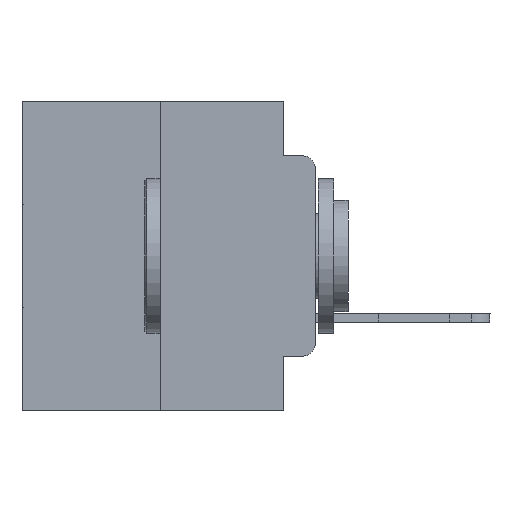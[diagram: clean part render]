
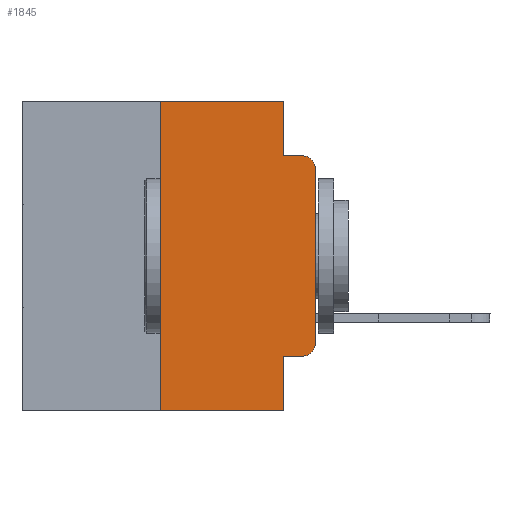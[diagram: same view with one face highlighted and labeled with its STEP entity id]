
A CAD part, left-side view. The second image highlights one B-rep face of the part: STEP entity #1845.
In plain terms, the highlighted planar face has unit normal (-1, 0, 0).
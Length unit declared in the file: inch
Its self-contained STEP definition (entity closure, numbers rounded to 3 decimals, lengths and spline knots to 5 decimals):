
#11 = VECTOR ( 'NONE', #9029, 39.37008 ) ;
#549 = ORIENTED_EDGE ( 'NONE', *, *, #20635, .T. ) ;
#1133 = VERTEX_POINT ( 'NONE', #3323 ) ;
#1257 = LINE ( 'NONE', #24410, #22145 ) ;
#1786 = CARTESIAN_POINT ( 'NONE',  ( 0., 0.02, -0.3915 ) ) ;
#1845 = ADVANCED_FACE ( 'NONE', ( #3311 ), #5530, .F. ) ;
#2125 = EDGE_CURVE ( 'NONE', #24953, #6071, #23184, .T. ) ;
#2326 = CARTESIAN_POINT ( 'NONE',  ( 0., 0.051, -0.0885 ) ) ;
#2658 = EDGE_CURVE ( 'NONE', #4916, #24879, #10917, .T. ) ;
#3274 = CARTESIAN_POINT ( 'NONE',  ( 0., 0.051, -0.5 ) ) ;
#3311 = FACE_OUTER_BOUND ( 'NONE', #5650, .T. ) ;
#3323 = CARTESIAN_POINT ( 'NONE',  ( 0., 0., -0.1085 ) ) ;
#3436 = CARTESIAN_POINT ( 'NONE',  ( 0., 0.051, 0. ) ) ;
#3917 = VERTEX_POINT ( 'NONE', #7481 ) ;
#4213 = CARTESIAN_POINT ( 'NONE',  ( 0., 0.473, 0. ) ) ;
#4224 = DIRECTION ( 'NONE',  ( 0., 0., 1. ) ) ;
#4415 = CARTESIAN_POINT ( 'NONE',  ( 0., 0., 0. ) ) ;
#4502 = CARTESIAN_POINT ( 'NONE',  ( 0., 0.02, -0.0885 ) ) ;
#4613 = EDGE_CURVE ( 'NONE', #24413, #24953, #23400, .T. ) ;
#4916 = VERTEX_POINT ( 'NONE', #19216 ) ;
#5120 = ORIENTED_EDGE ( 'NONE', *, *, #14701, .T. ) ;
#5386 = LINE ( 'NONE', #20365, #8354 ) ;
#5530 = PLANE ( 'NONE',  #8370 ) ;
#5650 = EDGE_LOOP ( 'NONE', ( #13415, #8074, #25949, #16573, #19299, #25915, #549, #20449, #17535, #5120 ) ) ;
#5832 = CIRCLE ( 'NONE', #15003, 0.02 ) ;
#6071 = VERTEX_POINT ( 'NONE', #3436 ) ;
#6528 = CIRCLE ( 'NONE', #19536, 0.02 ) ;
#6769 = VERTEX_POINT ( 'NONE', #2326 ) ;
#7481 = CARTESIAN_POINT ( 'NONE',  ( 0., 0.02, -0.4115 ) ) ;
#7547 = DIRECTION ( 'NONE',  ( 0., 0., -1. ) ) ;
#7846 = DIRECTION ( 'NONE',  ( 0., 0., -1. ) ) ;
#7897 = DIRECTION ( 'NONE',  ( -1., 0., 0. ) ) ;
#8070 = EDGE_CURVE ( 'NONE', #4916, #3917, #1257, .T. ) ;
#8074 = ORIENTED_EDGE ( 'NONE', *, *, #18147, .T. ) ;
#8200 = CARTESIAN_POINT ( 'NONE',  ( 0., 0.25, 0. ) ) ;
#8354 = VECTOR ( 'NONE', #7547, 39.37008 ) ;
#8370 = AXIS2_PLACEMENT_3D ( 'NONE', #14064, #20655, #7846 ) ;
#8768 = DIRECTION ( 'NONE',  ( 0., 0., -1. ) ) ;
#9029 = DIRECTION ( 'NONE',  ( 0., 0., -1. ) ) ;
#9088 = CARTESIAN_POINT ( 'NONE',  ( 0., 0., -0.3915 ) ) ;
#10396 = VECTOR ( 'NONE', #23461, 39.37008 ) ;
#10467 = VECTOR ( 'NONE', #21643, 39.37008 ) ;
#10805 = VECTOR ( 'NONE', #4224, 39.37008 ) ;
#10917 = LINE ( 'NONE', #19531, #11 ) ;
#11549 = CARTESIAN_POINT ( 'NONE',  ( 0., 0.25, -0.5 ) ) ;
#12240 = VECTOR ( 'NONE', #15158, 39.37008 ) ;
#12473 = LINE ( 'NONE', #4415, #10467 ) ;
#13415 = ORIENTED_EDGE ( 'NONE', *, *, #15674, .T. ) ;
#14064 = CARTESIAN_POINT ( 'NONE',  ( 0., 0.473, 0. ) ) ;
#14701 = EDGE_CURVE ( 'NONE', #3917, #21515, #5832, .T. ) ;
#15003 = AXIS2_PLACEMENT_3D ( 'NONE', #1786, #7897, #18744 ) ;
#15090 = DIRECTION ( 'NONE',  ( -1., 0., 0. ) ) ;
#15158 = DIRECTION ( 'NONE',  ( 0., -1., 0. ) ) ;
#15455 = CARTESIAN_POINT ( 'NONE',  ( 0., 0.02, -0.1085 ) ) ;
#15674 = EDGE_CURVE ( 'NONE', #21515, #1133, #12473, .T. ) ;
#15690 = DIRECTION ( 'NONE',  ( 0., -1., 0. ) ) ;
#16573 = ORIENTED_EDGE ( 'NONE', *, *, #22687, .F. ) ;
#16865 = LINE ( 'NONE', #25464, #12240 ) ;
#17535 = ORIENTED_EDGE ( 'NONE', *, *, #8070, .T. ) ;
#18147 = EDGE_CURVE ( 'NONE', #1133, #20610, #6528, .T. ) ;
#18744 = DIRECTION ( 'NONE',  ( 0., 0., -1. ) ) ;
#19216 = CARTESIAN_POINT ( 'NONE',  ( 0., 0.051, -0.4115 ) ) ;
#19299 = ORIENTED_EDGE ( 'NONE', *, *, #2125, .F. ) ;
#19531 = CARTESIAN_POINT ( 'NONE',  ( 0., 0.051, 0. ) ) ;
#19536 = AXIS2_PLACEMENT_3D ( 'NONE', #15455, #15090, #8768 ) ;
#20365 = CARTESIAN_POINT ( 'NONE',  ( 0., 0.051, 0. ) ) ;
#20449 = ORIENTED_EDGE ( 'NONE', *, *, #2658, .F. ) ;
#20610 = VERTEX_POINT ( 'NONE', #4502 ) ;
#20635 = EDGE_CURVE ( 'NONE', #24413, #24879, #16865, .T. ) ;
#20655 = DIRECTION ( 'NONE',  ( 1., 0., 0. ) ) ;
#21345 = EDGE_CURVE ( 'NONE', #6769, #20610, #26365, .T. ) ;
#21515 = VERTEX_POINT ( 'NONE', #9088 ) ;
#21643 = DIRECTION ( 'NONE',  ( 0., 0., 1. ) ) ;
#22145 = VECTOR ( 'NONE', #15690, 39.37008 ) ;
#22687 = EDGE_CURVE ( 'NONE', #6071, #6769, #5386, .T. ) ;
#22830 = CARTESIAN_POINT ( 'NONE',  ( 0., 0.25, 0. ) ) ;
#23184 = LINE ( 'NONE', #4213, #27223 ) ;
#23400 = LINE ( 'NONE', #8200, #10805 ) ;
#23461 = DIRECTION ( 'NONE',  ( 0., -1., 0. ) ) ;
#23744 = CARTESIAN_POINT ( 'NONE',  ( 0., 0.051, -0.0885 ) ) ;
#24410 = CARTESIAN_POINT ( 'NONE',  ( 0., 0.051, -0.4115 ) ) ;
#24413 = VERTEX_POINT ( 'NONE', #11549 ) ;
#24879 = VERTEX_POINT ( 'NONE', #3274 ) ;
#24953 = VERTEX_POINT ( 'NONE', #22830 ) ;
#25077 = DIRECTION ( 'NONE',  ( 0., -1., 0. ) ) ;
#25464 = CARTESIAN_POINT ( 'NONE',  ( 0., 0.473, -0.5 ) ) ;
#25915 = ORIENTED_EDGE ( 'NONE', *, *, #4613, .F. ) ;
#25949 = ORIENTED_EDGE ( 'NONE', *, *, #21345, .F. ) ;
#26365 = LINE ( 'NONE', #23744, #10396 ) ;
#27223 = VECTOR ( 'NONE', #25077, 39.37008 ) ;
